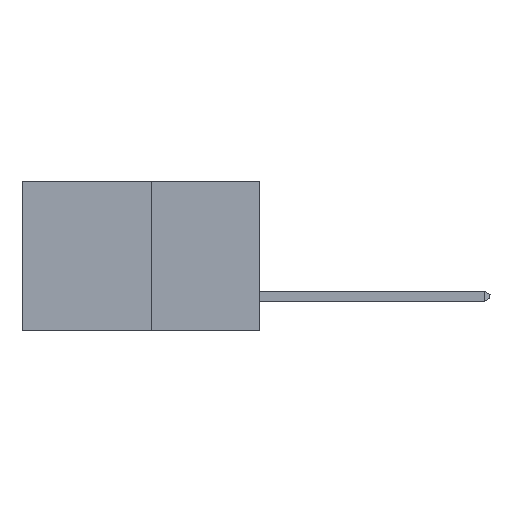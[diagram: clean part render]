
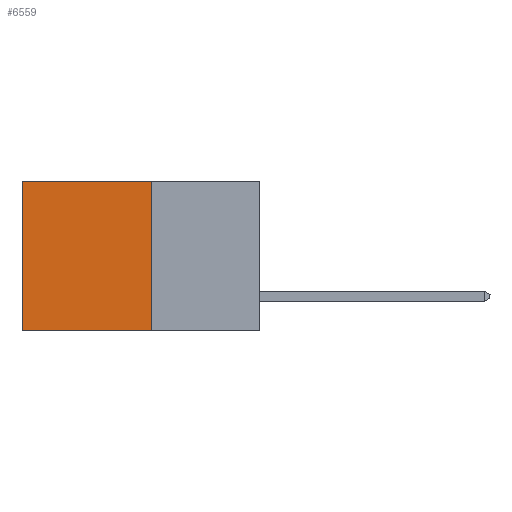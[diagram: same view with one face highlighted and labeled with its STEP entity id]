
A CAD part, left-side view. The second image highlights one B-rep face of the part: STEP entity #6559.
In plain terms, the highlighted planar face has unit normal (-1, 0, 0).
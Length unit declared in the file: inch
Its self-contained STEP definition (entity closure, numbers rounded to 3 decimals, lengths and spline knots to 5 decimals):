
#655 = EDGE_CURVE ( 'NONE', #15366, #2090, #2067, .T. ) ;
#1151 = VERTEX_POINT ( 'NONE', #8796 ) ;
#1607 = VECTOR ( 'NONE', #5100, 39.37008 ) ;
#2067 = LINE ( 'NONE', #12770, #1607 ) ;
#2090 = VERTEX_POINT ( 'NONE', #4578 ) ;
#2880 = EDGE_LOOP ( 'NONE', ( #6077, #11165, #12948, #18026 ) ) ;
#4048 = EDGE_CURVE ( 'NONE', #2090, #7969, #14682, .T. ) ;
#4081 = CARTESIAN_POINT ( 'NONE',  ( 0.277, 0.59, -0.37 ) ) ;
#4083 = PLANE ( 'NONE',  #11257 ) ;
#4395 = CARTESIAN_POINT ( 'NONE',  ( 0.277, 0.27, 0. ) ) ;
#4578 = CARTESIAN_POINT ( 'NONE',  ( 0.277, 0.59, 0. ) ) ;
#4723 = EDGE_CURVE ( 'NONE', #1151, #7969, #11145, .T. ) ;
#5100 = DIRECTION ( 'NONE',  ( 0., 1., 0. ) ) ;
#6077 = ORIENTED_EDGE ( 'NONE', *, *, #4048, .T. ) ;
#6559 = ADVANCED_FACE ( 'NONE', ( #9047 ), #4083, .F. ) ;
#6908 = VECTOR ( 'NONE', #10118, 39.37008 ) ;
#6956 = DIRECTION ( 'NONE',  ( 0., 0., -1. ) ) ;
#7171 = VECTOR ( 'NONE', #11760, 39.37008 ) ;
#7828 = VECTOR ( 'NONE', #10070, 39.37008 ) ;
#7969 = VERTEX_POINT ( 'NONE', #4081 ) ;
#8628 = CARTESIAN_POINT ( 'NONE',  ( 0.277, 0.27, -0.37 ) ) ;
#8796 = CARTESIAN_POINT ( 'NONE',  ( 0.277, 0.27, -0.37 ) ) ;
#9047 = FACE_OUTER_BOUND ( 'NONE', #2880, .T. ) ;
#10070 = DIRECTION ( 'NONE',  ( 0., 0., -1. ) ) ;
#10118 = DIRECTION ( 'NONE',  ( 0., 1., 0. ) ) ;
#11145 = LINE ( 'NONE', #11548, #6908 ) ;
#11165 = ORIENTED_EDGE ( 'NONE', *, *, #4723, .F. ) ;
#11257 = AXIS2_PLACEMENT_3D ( 'NONE', #13982, #15466, #6956 ) ;
#11548 = CARTESIAN_POINT ( 'NONE',  ( 0.277, 0.27, -0.37 ) ) ;
#11760 = DIRECTION ( 'NONE',  ( 0., 0., -1. ) ) ;
#12170 = CARTESIAN_POINT ( 'NONE',  ( 0.277, 0.59, -0.37 ) ) ;
#12770 = CARTESIAN_POINT ( 'NONE',  ( 0.277, 0.27, 0. ) ) ;
#12948 = ORIENTED_EDGE ( 'NONE', *, *, #14692, .F. ) ;
#13982 = CARTESIAN_POINT ( 'NONE',  ( 0.277, 0.27, -0.37 ) ) ;
#14682 = LINE ( 'NONE', #12170, #7171 ) ;
#14692 = EDGE_CURVE ( 'NONE', #15366, #1151, #15376, .T. ) ;
#15366 = VERTEX_POINT ( 'NONE', #4395 ) ;
#15376 = LINE ( 'NONE', #8628, #7828 ) ;
#15466 = DIRECTION ( 'NONE',  ( 1., 0., 0. ) ) ;
#18026 = ORIENTED_EDGE ( 'NONE', *, *, #655, .T. ) ;
